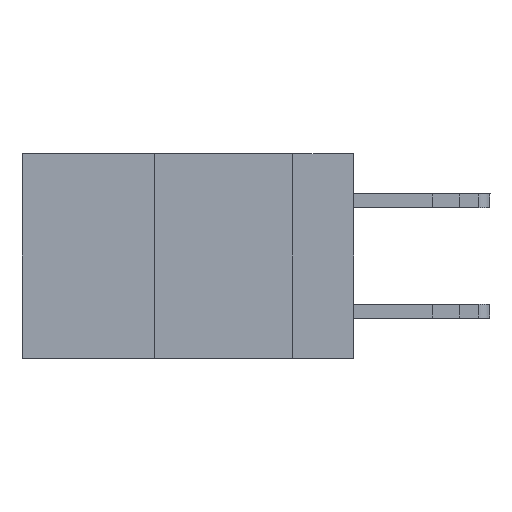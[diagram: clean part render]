
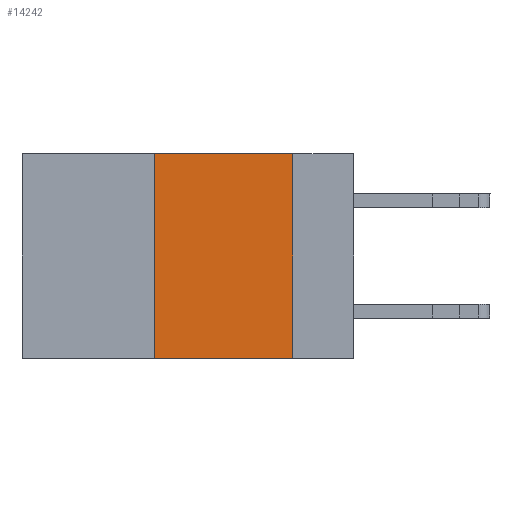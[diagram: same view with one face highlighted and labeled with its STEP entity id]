
A CAD part, left-side view. The second image highlights one B-rep face of the part: STEP entity #14242.
In plain terms, the highlighted planar face has unit normal (-1, 0, 0).
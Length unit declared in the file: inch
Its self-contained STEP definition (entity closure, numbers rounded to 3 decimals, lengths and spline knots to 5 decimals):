
#65 = LINE ( 'NONE', #2273, #10410 ) ;
#421 = PLANE ( 'NONE',  #10187 ) ;
#502 = DIRECTION ( 'NONE',  ( 1., 0., 0. ) ) ;
#1582 = CARTESIAN_POINT ( 'NONE',  ( 0., 0.36, 0. ) ) ;
#1875 = FACE_OUTER_BOUND ( 'NONE', #7565, .T. ) ;
#2113 = CARTESIAN_POINT ( 'NONE',  ( 0., 0.36, 0. ) ) ;
#2273 = CARTESIAN_POINT ( 'NONE',  ( 0., 0.6, 0. ) ) ;
#2342 = LINE ( 'NONE', #1582, #8196 ) ;
#2492 = CARTESIAN_POINT ( 'NONE',  ( 0., 0.11, -0.37 ) ) ;
#3296 = ORIENTED_EDGE ( 'NONE', *, *, #4226, .F. ) ;
#3535 = LINE ( 'NONE', #20217, #4641 ) ;
#4087 = CARTESIAN_POINT ( 'NONE',  ( 0., 0.6, 0. ) ) ;
#4145 = DIRECTION ( 'NONE',  ( 0., -1., 0. ) ) ;
#4226 = EDGE_CURVE ( 'NONE', #16020, #14863, #15262, .T. ) ;
#4413 = ORIENTED_EDGE ( 'NONE', *, *, #16612, .F. ) ;
#4641 = VECTOR ( 'NONE', #21949, 39.37008 ) ;
#5864 = DIRECTION ( 'NONE',  ( 0., 0., -1. ) ) ;
#5884 = ORIENTED_EDGE ( 'NONE', *, *, #16879, .F. ) ;
#7017 = DIRECTION ( 'NONE',  ( 0., 0., 1. ) ) ;
#7557 = EDGE_CURVE ( 'NONE', #22393, #14863, #3535, .T. ) ;
#7565 = EDGE_LOOP ( 'NONE', ( #3296, #5884, #4413, #23115 ) ) ;
#8196 = VECTOR ( 'NONE', #7017, 39.37008 ) ;
#10187 = AXIS2_PLACEMENT_3D ( 'NONE', #4087, #502, #5864 ) ;
#10410 = VECTOR ( 'NONE', #4145, 39.37008 ) ;
#11391 = DIRECTION ( 'NONE',  ( 0., 0., -1. ) ) ;
#12152 = VECTOR ( 'NONE', #11391, 39.37008 ) ;
#14242 = ADVANCED_FACE ( 'NONE', ( #1875 ), #421, .F. ) ;
#14863 = VERTEX_POINT ( 'NONE', #2492 ) ;
#15262 = LINE ( 'NONE', #18619, #12152 ) ;
#16020 = VERTEX_POINT ( 'NONE', #21059 ) ;
#16612 = EDGE_CURVE ( 'NONE', #22393, #18766, #2342, .T. ) ;
#16879 = EDGE_CURVE ( 'NONE', #18766, #16020, #65, .T. ) ;
#17827 = CARTESIAN_POINT ( 'NONE',  ( 0., 0.36, -0.37 ) ) ;
#18619 = CARTESIAN_POINT ( 'NONE',  ( 0., 0.11, 0. ) ) ;
#18766 = VERTEX_POINT ( 'NONE', #2113 ) ;
#20217 = CARTESIAN_POINT ( 'NONE',  ( 0., 0.6, -0.37 ) ) ;
#21059 = CARTESIAN_POINT ( 'NONE',  ( 0., 0.11, 0. ) ) ;
#21949 = DIRECTION ( 'NONE',  ( 0., -1., 0. ) ) ;
#22393 = VERTEX_POINT ( 'NONE', #17827 ) ;
#23115 = ORIENTED_EDGE ( 'NONE', *, *, #7557, .T. ) ;
